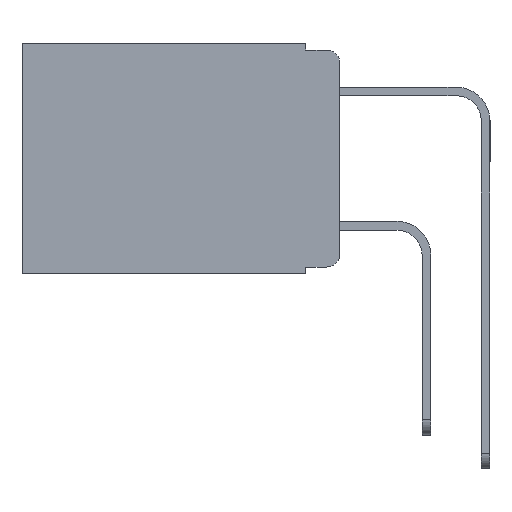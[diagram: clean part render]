
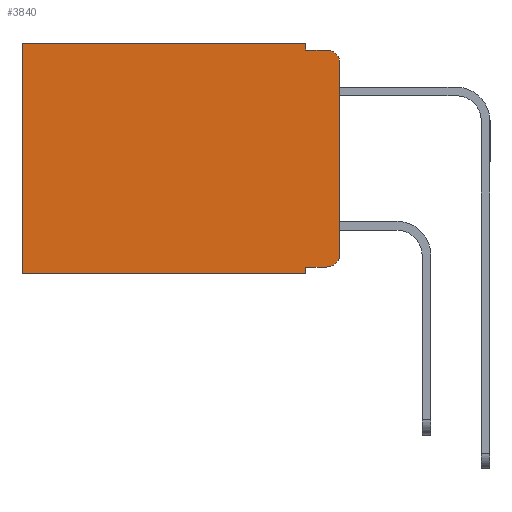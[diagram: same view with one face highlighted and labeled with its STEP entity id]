
A CAD part, left-side view. The second image highlights one B-rep face of the part: STEP entity #3840.
In plain terms, the highlighted planar face has unit normal (-1, 0, 0).
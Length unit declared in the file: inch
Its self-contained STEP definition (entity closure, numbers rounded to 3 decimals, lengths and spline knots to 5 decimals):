
#128 = CIRCLE ( 'NONE', #8893, 0.02 ) ;
#131 = CARTESIAN_POINT ( 'NONE',  ( 0.298, 0.473, -0.343 ) ) ;
#274 = ORIENTED_EDGE ( 'NONE', *, *, #4051, .T. ) ;
#366 = ORIENTED_EDGE ( 'NONE', *, *, #4348, .T. ) ;
#434 = DIRECTION ( 'NONE',  ( 0., 1., 0. ) ) ;
#699 = EDGE_CURVE ( 'NONE', #12644, #3252, #14075, .T. ) ;
#1047 = VECTOR ( 'NONE', #5067, 39.37008 ) ;
#1116 = VERTEX_POINT ( 'NONE', #1695 ) ;
#1425 = LINE ( 'NONE', #7489, #1047 ) ;
#1646 = EDGE_CURVE ( 'NONE', #2820, #4449, #8353, .T. ) ;
#1695 = CARTESIAN_POINT ( 'NONE',  ( 0.298, 0.02, -0.333 ) ) ;
#2177 = ORIENTED_EDGE ( 'NONE', *, *, #4987, .F. ) ;
#2607 = AXIS2_PLACEMENT_3D ( 'NONE', #11885, #10715, #10443 ) ;
#2802 = LINE ( 'NONE', #6346, #10814 ) ;
#2803 = CARTESIAN_POINT ( 'NONE',  ( 0.298, 0.051, -0.333 ) ) ;
#2820 = VERTEX_POINT ( 'NONE', #4818 ) ;
#2926 = ORIENTED_EDGE ( 'NONE', *, *, #7380, .T. ) ;
#2945 = CARTESIAN_POINT ( 'NONE',  ( 0.298, 0.02, -0.03 ) ) ;
#3022 = LINE ( 'NONE', #12392, #5713 ) ;
#3252 = VERTEX_POINT ( 'NONE', #7298 ) ;
#3322 = ORIENTED_EDGE ( 'NONE', *, *, #5502, .T. ) ;
#3840 = ADVANCED_FACE ( 'NONE', ( #13671 ), #6096, .F. ) ;
#4051 = EDGE_CURVE ( 'NONE', #1116, #3252, #11065, .T. ) ;
#4152 = VERTEX_POINT ( 'NONE', #2803 ) ;
#4235 = ORIENTED_EDGE ( 'NONE', *, *, #699, .F. ) ;
#4348 = EDGE_CURVE ( 'NONE', #4152, #1116, #1425, .T. ) ;
#4449 = VERTEX_POINT ( 'NONE', #10056 ) ;
#4644 = VERTEX_POINT ( 'NONE', #12206 ) ;
#4762 = VERTEX_POINT ( 'NONE', #131 ) ;
#4818 = CARTESIAN_POINT ( 'NONE',  ( 0.298, 0.051, 0. ) ) ;
#4900 = VECTOR ( 'NONE', #8068, 39.37008 ) ;
#4906 = CARTESIAN_POINT ( 'NONE',  ( 0.298, 0.051, 0. ) ) ;
#4914 = LINE ( 'NONE', #4906, #7662 ) ;
#4987 = EDGE_CURVE ( 'NONE', #4449, #6529, #3022, .T. ) ;
#5067 = DIRECTION ( 'NONE',  ( 0., -1., 0. ) ) ;
#5502 = EDGE_CURVE ( 'NONE', #12644, #6529, #128, .T. ) ;
#5642 = DIRECTION ( 'NONE',  ( 0., 0., -1. ) ) ;
#5713 = VECTOR ( 'NONE', #12463, 39.37008 ) ;
#5990 = DIRECTION ( 'NONE',  ( 0., 0., -1. ) ) ;
#6063 = CARTESIAN_POINT ( 'NONE',  ( 0.298, 0., -0.343 ) ) ;
#6089 = DIRECTION ( 'NONE',  ( 0., 0., -1. ) ) ;
#6096 = PLANE ( 'NONE',  #9791 ) ;
#6233 = LINE ( 'NONE', #9631, #8929 ) ;
#6309 = DIRECTION ( 'NONE',  ( 0., 0., -1. ) ) ;
#6346 = CARTESIAN_POINT ( 'NONE',  ( 0.298, 0.473, 0. ) ) ;
#6447 = EDGE_LOOP ( 'NONE', ( #4235, #3322, #2177, #9609, #2926, #8692, #9191, #13298, #366, #274 ) ) ;
#6479 = DIRECTION ( 'NONE',  ( -1., 0., 0. ) ) ;
#6529 = VERTEX_POINT ( 'NONE', #9308 ) ;
#7075 = VERTEX_POINT ( 'NONE', #13303 ) ;
#7298 = CARTESIAN_POINT ( 'NONE',  ( 0.298, 0., -0.313 ) ) ;
#7380 = EDGE_CURVE ( 'NONE', #2820, #7075, #6233, .T. ) ;
#7465 = EDGE_CURVE ( 'NONE', #7075, #4762, #2802, .T. ) ;
#7489 = CARTESIAN_POINT ( 'NONE',  ( 0.298, 0.051, -0.333 ) ) ;
#7525 = DIRECTION ( 'NONE',  ( 0., 0., -1. ) ) ;
#7662 = VECTOR ( 'NONE', #6089, 39.37008 ) ;
#7995 = CARTESIAN_POINT ( 'NONE',  ( 0.298, 0., -0.03 ) ) ;
#8068 = DIRECTION ( 'NONE',  ( 0., 0., -1. ) ) ;
#8285 = VECTOR ( 'NONE', #10603, 39.37008 ) ;
#8353 = LINE ( 'NONE', #11952, #4900 ) ;
#8643 = LINE ( 'NONE', #6063, #8285 ) ;
#8692 = ORIENTED_EDGE ( 'NONE', *, *, #7465, .T. ) ;
#8893 = AXIS2_PLACEMENT_3D ( 'NONE', #2945, #6479, #5990 ) ;
#8929 = VECTOR ( 'NONE', #434, 39.37008 ) ;
#9191 = ORIENTED_EDGE ( 'NONE', *, *, #12840, .F. ) ;
#9308 = CARTESIAN_POINT ( 'NONE',  ( 0.298, 0.02, -0.01 ) ) ;
#9609 = ORIENTED_EDGE ( 'NONE', *, *, #1646, .F. ) ;
#9631 = CARTESIAN_POINT ( 'NONE',  ( 0.298, 0., 0. ) ) ;
#9754 = EDGE_CURVE ( 'NONE', #4152, #4644, #4914, .T. ) ;
#9791 = AXIS2_PLACEMENT_3D ( 'NONE', #13020, #13098, #6309 ) ;
#10056 = CARTESIAN_POINT ( 'NONE',  ( 0.298, 0.051, -0.01 ) ) ;
#10443 = DIRECTION ( 'NONE',  ( 0., 0., -1. ) ) ;
#10603 = DIRECTION ( 'NONE',  ( 0., 1., 0. ) ) ;
#10715 = DIRECTION ( 'NONE',  ( -1., 0., 0. ) ) ;
#10791 = CARTESIAN_POINT ( 'NONE',  ( 0.298, 0., 0. ) ) ;
#10814 = VECTOR ( 'NONE', #7525, 39.37008 ) ;
#11065 = CIRCLE ( 'NONE', #2607, 0.02 ) ;
#11328 = VECTOR ( 'NONE', #5642, 39.37008 ) ;
#11885 = CARTESIAN_POINT ( 'NONE',  ( 0.298, 0.02, -0.313 ) ) ;
#11952 = CARTESIAN_POINT ( 'NONE',  ( 0.298, 0.051, 0. ) ) ;
#12206 = CARTESIAN_POINT ( 'NONE',  ( 0.298, 0.051, -0.343 ) ) ;
#12392 = CARTESIAN_POINT ( 'NONE',  ( 0.298, 0.051, -0.01 ) ) ;
#12463 = DIRECTION ( 'NONE',  ( 0., -1., 0. ) ) ;
#12644 = VERTEX_POINT ( 'NONE', #7995 ) ;
#12840 = EDGE_CURVE ( 'NONE', #4644, #4762, #8643, .T. ) ;
#13020 = CARTESIAN_POINT ( 'NONE',  ( 0.298, 0., 0. ) ) ;
#13098 = DIRECTION ( 'NONE',  ( 1., 0., 0. ) ) ;
#13298 = ORIENTED_EDGE ( 'NONE', *, *, #9754, .F. ) ;
#13303 = CARTESIAN_POINT ( 'NONE',  ( 0.298, 0.473, 0. ) ) ;
#13671 = FACE_OUTER_BOUND ( 'NONE', #6447, .T. ) ;
#14075 = LINE ( 'NONE', #10791, #11328 ) ;
